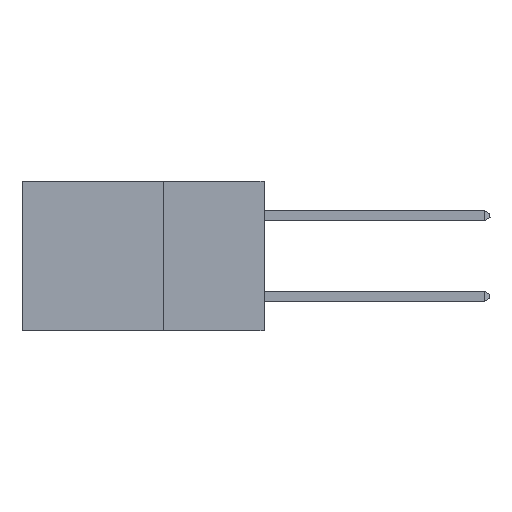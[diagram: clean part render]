
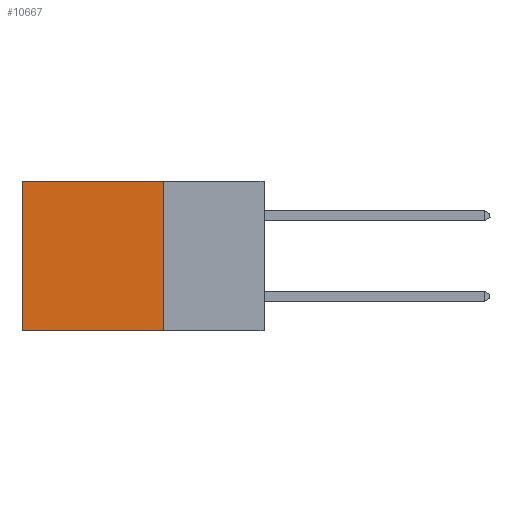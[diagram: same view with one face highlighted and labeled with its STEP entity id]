
A CAD part, left-side view. The second image highlights one B-rep face of the part: STEP entity #10667.
In plain terms, the highlighted planar face has unit normal (-1, 0, 0).
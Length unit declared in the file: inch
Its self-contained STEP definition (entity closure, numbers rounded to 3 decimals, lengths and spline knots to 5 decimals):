
#741 = CARTESIAN_POINT ( 'NONE',  ( 0.298, 0.25, -0.37 ) ) ;
#1975 = VECTOR ( 'NONE', #27287, 39.37008 ) ;
#2064 = CARTESIAN_POINT ( 'NONE',  ( 0.298, 0.25, 0. ) ) ;
#2197 = AXIS2_PLACEMENT_3D ( 'NONE', #2064, #4309, #16140 ) ;
#2733 = CARTESIAN_POINT ( 'NONE',  ( 0.298, 0.25, 0. ) ) ;
#3307 = CARTESIAN_POINT ( 'NONE',  ( 0.298, 0.6, 0. ) ) ;
#4309 = DIRECTION ( 'NONE',  ( 1., 0., 0. ) ) ;
#4515 = FACE_OUTER_BOUND ( 'NONE', #28535, .T. ) ;
#6110 = ORIENTED_EDGE ( 'NONE', *, *, #11750, .T. ) ;
#6895 = LINE ( 'NONE', #3307, #21556 ) ;
#7848 = DIRECTION ( 'NONE',  ( 0., 0., -1. ) ) ;
#8016 = VERTEX_POINT ( 'NONE', #11823 ) ;
#8347 = LINE ( 'NONE', #22764, #1975 ) ;
#10265 = ORIENTED_EDGE ( 'NONE', *, *, #12793, .F. ) ;
#10568 = VECTOR ( 'NONE', #19003, 39.37008 ) ;
#10667 = ADVANCED_FACE ( 'NONE', ( #4515 ), #26936, .F. ) ;
#11750 = EDGE_CURVE ( 'NONE', #23453, #25562, #6895, .T. ) ;
#11823 = CARTESIAN_POINT ( 'NONE',  ( 0.298, 0.25, 0. ) ) ;
#12618 = ORIENTED_EDGE ( 'NONE', *, *, #29049, .F. ) ;
#12793 = EDGE_CURVE ( 'NONE', #8016, #20776, #23212, .T. ) ;
#14373 = CARTESIAN_POINT ( 'NONE',  ( 0.298, 0.6, 0. ) ) ;
#16140 = DIRECTION ( 'NONE',  ( 0., 0., -1. ) ) ;
#16741 = ORIENTED_EDGE ( 'NONE', *, *, #21161, .T. ) ;
#17221 = CARTESIAN_POINT ( 'NONE',  ( 0.298, 0.6, -0.37 ) ) ;
#19003 = DIRECTION ( 'NONE',  ( 0., 1., 0. ) ) ;
#20776 = VERTEX_POINT ( 'NONE', #741 ) ;
#21161 = EDGE_CURVE ( 'NONE', #8016, #23453, #24092, .T. ) ;
#21556 = VECTOR ( 'NONE', #7848, 39.37008 ) ;
#22764 = CARTESIAN_POINT ( 'NONE',  ( 0.298, 0.25, -0.37 ) ) ;
#22820 = CARTESIAN_POINT ( 'NONE',  ( 0.298, 0.25, 0. ) ) ;
#23087 = DIRECTION ( 'NONE',  ( 0., 0., -1. ) ) ;
#23212 = LINE ( 'NONE', #22820, #23555 ) ;
#23453 = VERTEX_POINT ( 'NONE', #14373 ) ;
#23555 = VECTOR ( 'NONE', #23087, 39.37008 ) ;
#24092 = LINE ( 'NONE', #2733, #10568 ) ;
#25562 = VERTEX_POINT ( 'NONE', #17221 ) ;
#26936 = PLANE ( 'NONE',  #2197 ) ;
#27287 = DIRECTION ( 'NONE',  ( 0., 1., 0. ) ) ;
#28535 = EDGE_LOOP ( 'NONE', ( #6110, #12618, #10265, #16741 ) ) ;
#29049 = EDGE_CURVE ( 'NONE', #20776, #25562, #8347, .T. ) ;
